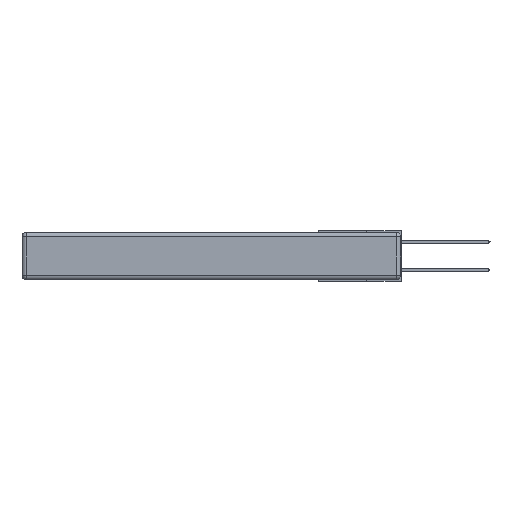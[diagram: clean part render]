
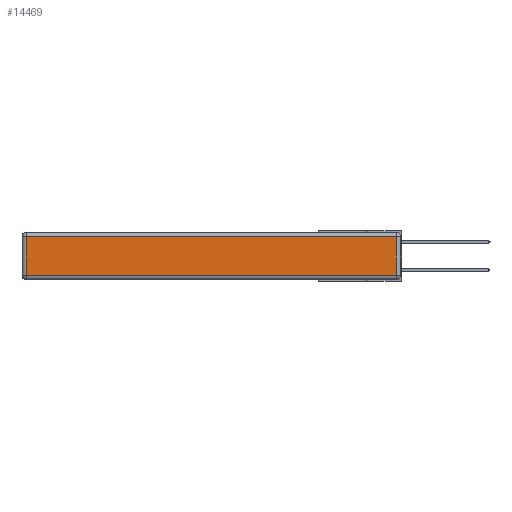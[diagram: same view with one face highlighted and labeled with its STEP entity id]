
A CAD part, left-side view. The second image highlights one B-rep face of the part: STEP entity #14469.
In plain terms, the highlighted planar face has unit normal (-1, 0, 0).
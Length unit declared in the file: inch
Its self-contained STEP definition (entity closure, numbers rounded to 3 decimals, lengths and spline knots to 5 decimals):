
#1914 = ORIENTED_EDGE ( 'NONE', *, *, #7062, .T. ) ;
#1953 = EDGE_CURVE ( 'NONE', #3358, #7152, #9753, .T. ) ;
#2707 = FACE_OUTER_BOUND ( 'NONE', #4375, .T. ) ;
#3349 = EDGE_CURVE ( 'NONE', #6515, #3358, #13620, .T. ) ;
#3358 = VERTEX_POINT ( 'NONE', #15294 ) ;
#4306 = DIRECTION ( 'NONE',  ( 0., 0., -1. ) ) ;
#4375 = EDGE_LOOP ( 'NONE', ( #9212, #4719, #12096, #1914 ) ) ;
#4380 = DIRECTION ( 'NONE',  ( -1., 0., 0. ) ) ;
#4719 = ORIENTED_EDGE ( 'NONE', *, *, #3349, .T. ) ;
#5335 = DIRECTION ( 'NONE',  ( 0., 0., 1. ) ) ;
#5369 = DIRECTION ( 'NONE',  ( 0., -1., 0. ) ) ;
#5570 = VECTOR ( 'NONE', #5369, 39.37008 ) ;
#6045 = VERTEX_POINT ( 'NONE', #11364 ) ;
#6360 = CARTESIAN_POINT ( 'NONE',  ( 0., 2.75, -0.03 ) ) ;
#6515 = VERTEX_POINT ( 'NONE', #10880 ) ;
#6847 = LINE ( 'NONE', #12408, #5570 ) ;
#7062 = EDGE_CURVE ( 'NONE', #7152, #6045, #8807, .T. ) ;
#7152 = VERTEX_POINT ( 'NONE', #14154 ) ;
#7182 = AXIS2_PLACEMENT_3D ( 'NONE', #14808, #4380, #5335 ) ;
#7758 = VECTOR ( 'NONE', #15183, 39.37008 ) ;
#8807 = LINE ( 'NONE', #10281, #12846 ) ;
#9212 = ORIENTED_EDGE ( 'NONE', *, *, #11488, .T. ) ;
#9753 = LINE ( 'NONE', #6360, #15324 ) ;
#10281 = CARTESIAN_POINT ( 'NONE',  ( 0., 2.72, -0.343 ) ) ;
#10880 = CARTESIAN_POINT ( 'NONE',  ( 0., 0.03, -0.313 ) ) ;
#11364 = CARTESIAN_POINT ( 'NONE',  ( 0., 2.72, -0.313 ) ) ;
#11488 = EDGE_CURVE ( 'NONE', #6045, #6515, #6847, .T. ) ;
#12096 = ORIENTED_EDGE ( 'NONE', *, *, #1953, .T. ) ;
#12408 = CARTESIAN_POINT ( 'NONE',  ( 0., 0., -0.313 ) ) ;
#12776 = CARTESIAN_POINT ( 'NONE',  ( 0., 0.03, -0.343 ) ) ;
#12846 = VECTOR ( 'NONE', #4306, 39.37008 ) ;
#13620 = LINE ( 'NONE', #12776, #7758 ) ;
#14154 = CARTESIAN_POINT ( 'NONE',  ( 0., 2.72, -0.03 ) ) ;
#14469 = ADVANCED_FACE ( 'NONE', ( #2707 ), #14971, .T. ) ;
#14596 = DIRECTION ( 'NONE',  ( 0., 1., 0. ) ) ;
#14808 = CARTESIAN_POINT ( 'NONE',  ( 0., 0., -0.343 ) ) ;
#14971 = PLANE ( 'NONE',  #7182 ) ;
#15183 = DIRECTION ( 'NONE',  ( 0., 0., 1. ) ) ;
#15294 = CARTESIAN_POINT ( 'NONE',  ( 0., 0.03, -0.03 ) ) ;
#15324 = VECTOR ( 'NONE', #14596, 39.37008 ) ;
